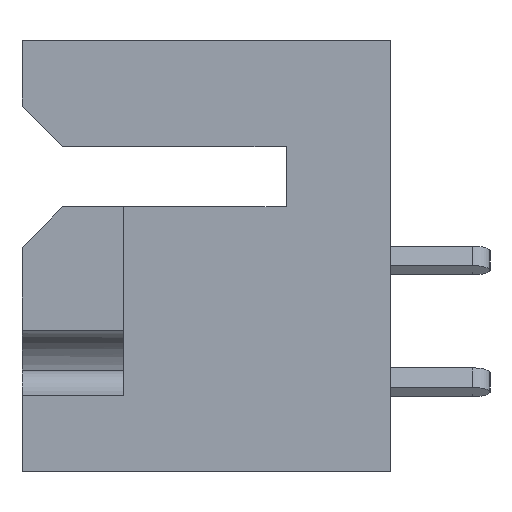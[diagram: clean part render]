
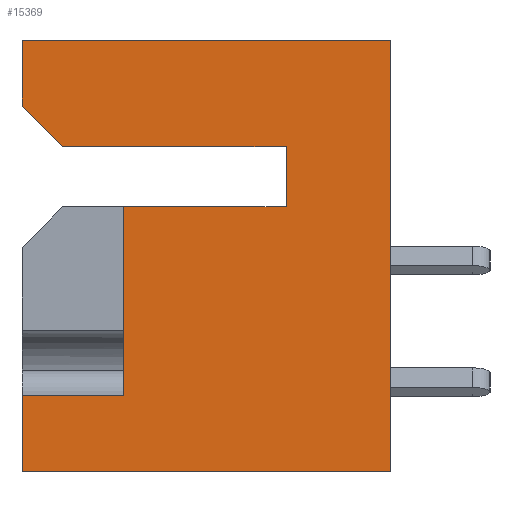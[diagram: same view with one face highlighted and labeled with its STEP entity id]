
A CAD part, left-side view. The second image highlights one B-rep face of the part: STEP entity #15369.
In plain terms, the highlighted planar face has unit normal (-1, 0, 0).
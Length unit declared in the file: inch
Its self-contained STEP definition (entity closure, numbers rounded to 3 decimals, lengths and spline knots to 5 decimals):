
#97 = DIRECTION ( 'NONE',  ( 0., -0.707, -0.707 ) ) ;
#432 = VECTOR ( 'NONE', #9249, 39.37008 ) ;
#759 = LINE ( 'NONE', #9492, #18542 ) ;
#900 = DIRECTION ( 'NONE',  ( 0., 0., 1. ) ) ;
#946 = CARTESIAN_POINT ( 'NONE',  ( 0., 0.453, 0. ) ) ;
#1275 = DIRECTION ( 'NONE',  ( 0., 0., 1. ) ) ;
#1322 = CARTESIAN_POINT ( 'NONE',  ( 0., 0.128, -0.131 ) ) ;
#1705 = CARTESIAN_POINT ( 'NONE',  ( 0., 0.128, -0.131 ) ) ;
#1827 = VECTOR ( 'NONE', #7890, 39.37008 ) ;
#1946 = FACE_OUTER_BOUND ( 'NONE', #7051, .T. ) ;
#1954 = CARTESIAN_POINT ( 'NONE',  ( 0., 0.453, -0.531 ) ) ;
#1964 = VERTEX_POINT ( 'NONE', #16801 ) ;
#2175 = DIRECTION ( 'NONE',  ( 0., 1., 0. ) ) ;
#2182 = VERTEX_POINT ( 'NONE', #12029 ) ;
#2732 = ORIENTED_EDGE ( 'NONE', *, *, #11893, .T. ) ;
#2993 = ORIENTED_EDGE ( 'NONE', *, *, #4269, .F. ) ;
#3051 = DIRECTION ( 'NONE',  ( 0., 0., 1. ) ) ;
#3178 = VECTOR ( 'NONE', #17451, 39.37008 ) ;
#3491 = DIRECTION ( 'NONE',  ( 1., 0., 0. ) ) ;
#3743 = CARTESIAN_POINT ( 'NONE',  ( 0., 0.128, -0.205 ) ) ;
#3759 = LINE ( 'NONE', #13432, #7287 ) ;
#4113 = LINE ( 'NONE', #16215, #17300 ) ;
#4269 = EDGE_CURVE ( 'NONE', #2182, #16595, #4870, .T. ) ;
#4870 = LINE ( 'NONE', #946, #17495 ) ;
#4935 = CARTESIAN_POINT ( 'NONE',  ( 0., 0.453, -0.437 ) ) ;
#4947 = ORIENTED_EDGE ( 'NONE', *, *, #20810, .T. ) ;
#5162 = AXIS2_PLACEMENT_3D ( 'NONE', #13805, #3491, #12742 ) ;
#5189 = EDGE_CURVE ( 'NONE', #16141, #1964, #18576, .T. ) ;
#5387 = VECTOR ( 'NONE', #1275, 39.37008 ) ;
#5530 = ORIENTED_EDGE ( 'NONE', *, *, #5189, .T. ) ;
#5596 = VECTOR ( 'NONE', #2175, 39.37008 ) ;
#5797 = CARTESIAN_POINT ( 'NONE',  ( 0., 0.128, -0.205 ) ) ;
#5924 = EDGE_CURVE ( 'NONE', #16595, #1964, #6709, .T. ) ;
#6334 = CARTESIAN_POINT ( 'NONE',  ( 0., 0., -0.531 ) ) ;
#6675 = LINE ( 'NONE', #5797, #432 ) ;
#6709 = LINE ( 'NONE', #11382, #1827 ) ;
#7051 = EDGE_LOOP ( 'NONE', ( #19136, #12962, #4947, #5530, #13273, #2993, #2732, #12117, #15518, #20893, #15026 ) ) ;
#7267 = VERTEX_POINT ( 'NONE', #7468 ) ;
#7287 = VECTOR ( 'NONE', #3051, 39.37008 ) ;
#7427 = VECTOR ( 'NONE', #11611, 39.37008 ) ;
#7468 = CARTESIAN_POINT ( 'NONE',  ( 0., 0.328, -0.205 ) ) ;
#7528 = VERTEX_POINT ( 'NONE', #1705 ) ;
#7890 = DIRECTION ( 'NONE',  ( 0., -1., 0. ) ) ;
#7897 = DIRECTION ( 'NONE',  ( 0., 0., 1. ) ) ;
#8324 = VERTEX_POINT ( 'NONE', #11071 ) ;
#9249 = DIRECTION ( 'NONE',  ( 0., 1., 0. ) ) ;
#9492 = CARTESIAN_POINT ( 'NONE',  ( 0., 0.453, 0. ) ) ;
#9624 = LINE ( 'NONE', #21173, #5596 ) ;
#10684 = VERTEX_POINT ( 'NONE', #15211 ) ;
#10823 = EDGE_CURVE ( 'NONE', #10684, #13862, #759, .T. ) ;
#11071 = CARTESIAN_POINT ( 'NONE',  ( 0., 0.328, -0.437 ) ) ;
#11122 = CARTESIAN_POINT ( 'NONE',  ( 0., 0.453, 0. ) ) ;
#11310 = EDGE_CURVE ( 'NONE', #8324, #13862, #9624, .T. ) ;
#11382 = CARTESIAN_POINT ( 'NONE',  ( 0., 0.453, 0. ) ) ;
#11611 = DIRECTION ( 'NONE',  ( 0., 1., 0. ) ) ;
#11718 = LINE ( 'NONE', #1322, #7427 ) ;
#11893 = EDGE_CURVE ( 'NONE', #2182, #19116, #21674, .T. ) ;
#12029 = CARTESIAN_POINT ( 'NONE',  ( 0., 0.453, -0.081 ) ) ;
#12117 = ORIENTED_EDGE ( 'NONE', *, *, #13771, .F. ) ;
#12742 = DIRECTION ( 'NONE',  ( 0., 0., -1. ) ) ;
#12962 = ORIENTED_EDGE ( 'NONE', *, *, #10823, .F. ) ;
#12982 = DIRECTION ( 'NONE',  ( 0., 0., 1. ) ) ;
#13273 = ORIENTED_EDGE ( 'NONE', *, *, #5924, .F. ) ;
#13432 = CARTESIAN_POINT ( 'NONE',  ( 0., 0.328, -0.205 ) ) ;
#13771 = EDGE_CURVE ( 'NONE', #7528, #19116, #11718, .T. ) ;
#13805 = CARTESIAN_POINT ( 'NONE',  ( 0., 0.453, 0. ) ) ;
#13862 = VERTEX_POINT ( 'NONE', #4935 ) ;
#15026 = ORIENTED_EDGE ( 'NONE', *, *, #17373, .F. ) ;
#15211 = CARTESIAN_POINT ( 'NONE',  ( 0., 0.453, -0.531 ) ) ;
#15271 = LINE ( 'NONE', #1954, #3178 ) ;
#15369 = ADVANCED_FACE ( 'NONE', ( #1946 ), #21304, .F. ) ;
#15489 = EDGE_CURVE ( 'NONE', #17065, #7528, #4113, .T. ) ;
#15518 = ORIENTED_EDGE ( 'NONE', *, *, #15489, .F. ) ;
#16141 = VERTEX_POINT ( 'NONE', #6334 ) ;
#16215 = CARTESIAN_POINT ( 'NONE',  ( 0., 0.128, -0.131 ) ) ;
#16595 = VERTEX_POINT ( 'NONE', #11122 ) ;
#16801 = CARTESIAN_POINT ( 'NONE',  ( 0., 0., 0. ) ) ;
#17065 = VERTEX_POINT ( 'NONE', #3743 ) ;
#17300 = VECTOR ( 'NONE', #7897, 39.37008 ) ;
#17373 = EDGE_CURVE ( 'NONE', #8324, #7267, #3759, .T. ) ;
#17451 = DIRECTION ( 'NONE',  ( 0., -1., 0. ) ) ;
#17495 = VECTOR ( 'NONE', #12982, 39.37008 ) ;
#18542 = VECTOR ( 'NONE', #900, 39.37008 ) ;
#18576 = LINE ( 'NONE', #18716, #5387 ) ;
#18716 = CARTESIAN_POINT ( 'NONE',  ( 0., 0., 0. ) ) ;
#19116 = VERTEX_POINT ( 'NONE', #21540 ) ;
#19136 = ORIENTED_EDGE ( 'NONE', *, *, #11310, .T. ) ;
#20697 = CARTESIAN_POINT ( 'NONE',  ( 0., 0.403, -0.131 ) ) ;
#20810 = EDGE_CURVE ( 'NONE', #10684, #16141, #15271, .T. ) ;
#20893 = ORIENTED_EDGE ( 'NONE', *, *, #20940, .T. ) ;
#20940 = EDGE_CURVE ( 'NONE', #17065, #7267, #6675, .T. ) ;
#21173 = CARTESIAN_POINT ( 'NONE',  ( 0., 0.328, -0.437 ) ) ;
#21304 = PLANE ( 'NONE',  #5162 ) ;
#21540 = CARTESIAN_POINT ( 'NONE',  ( 0., 0.403, -0.131 ) ) ;
#21674 = LINE ( 'NONE', #20697, #22219 ) ;
#22219 = VECTOR ( 'NONE', #97, 39.37008 ) ;
